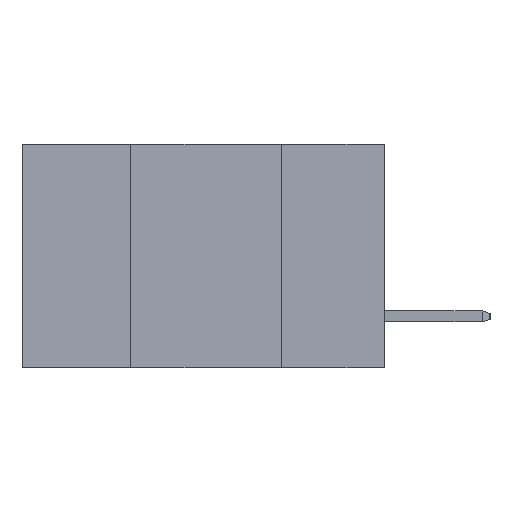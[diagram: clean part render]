
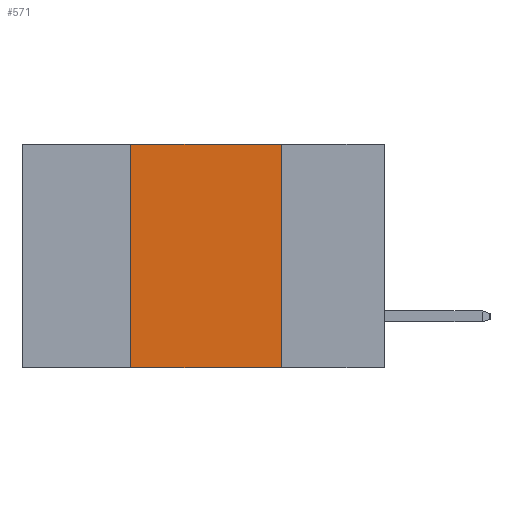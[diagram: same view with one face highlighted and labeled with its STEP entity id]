
A CAD part, left-side view. The second image highlights one B-rep face of the part: STEP entity #571.
In plain terms, the highlighted planar face has unit normal (-1, 0, 0).
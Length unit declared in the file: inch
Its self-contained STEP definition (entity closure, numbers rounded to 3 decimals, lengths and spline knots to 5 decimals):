
#571 = ADVANCED_FACE ( 'NONE', ( #13903 ), #10935, .F. ) ;
#1163 = VECTOR ( 'NONE', #1504, 39.37008 ) ;
#1504 = DIRECTION ( 'NONE',  ( 0., -1., 0. ) ) ;
#1578 = CARTESIAN_POINT ( 'NONE',  ( 0., 0.6, -0.37 ) ) ;
#1893 = DIRECTION ( 'NONE',  ( 0., -1., 0. ) ) ;
#2211 = CARTESIAN_POINT ( 'NONE',  ( 0., 0.17, -0.37 ) ) ;
#2545 = CARTESIAN_POINT ( 'NONE',  ( 0., 0.6, 0. ) ) ;
#3433 = CARTESIAN_POINT ( 'NONE',  ( 0., 0.42, -0.37 ) ) ;
#3455 = DIRECTION ( 'NONE',  ( 0., 0., 1. ) ) ;
#4135 = EDGE_CURVE ( 'NONE', #6457, #13559, #14386, .T. ) ;
#4667 = CARTESIAN_POINT ( 'NONE',  ( 0., 0.42, 0. ) ) ;
#4885 = CARTESIAN_POINT ( 'NONE',  ( 0., 0.6, 0. ) ) ;
#5698 = DIRECTION ( 'NONE',  ( 0., 0., -1. ) ) ;
#5726 = LINE ( 'NONE', #1578, #1163 ) ;
#6457 = VERTEX_POINT ( 'NONE', #4667 ) ;
#6764 = LINE ( 'NONE', #19108, #19841 ) ;
#6936 = VERTEX_POINT ( 'NONE', #18076 ) ;
#7564 = EDGE_LOOP ( 'NONE', ( #8768, #15022, #21575, #13736 ) ) ;
#8113 = EDGE_CURVE ( 'NONE', #6936, #6457, #21948, .T. ) ;
#8383 = DIRECTION ( 'NONE',  ( 1., 0., 0. ) ) ;
#8530 = VECTOR ( 'NONE', #3455, 39.37008 ) ;
#8768 = ORIENTED_EDGE ( 'NONE', *, *, #10841, .F. ) ;
#9779 = VECTOR ( 'NONE', #1893, 39.37008 ) ;
#10447 = EDGE_CURVE ( 'NONE', #6936, #15133, #5726, .T. ) ;
#10841 = EDGE_CURVE ( 'NONE', #13559, #15133, #6764, .T. ) ;
#10935 = PLANE ( 'NONE',  #12965 ) ;
#12965 = AXIS2_PLACEMENT_3D ( 'NONE', #4885, #8383, #5698 ) ;
#13559 = VERTEX_POINT ( 'NONE', #13832 ) ;
#13736 = ORIENTED_EDGE ( 'NONE', *, *, #10447, .T. ) ;
#13832 = CARTESIAN_POINT ( 'NONE',  ( 0., 0.17, 0. ) ) ;
#13903 = FACE_OUTER_BOUND ( 'NONE', #7564, .T. ) ;
#14386 = LINE ( 'NONE', #2545, #9779 ) ;
#15022 = ORIENTED_EDGE ( 'NONE', *, *, #4135, .F. ) ;
#15133 = VERTEX_POINT ( 'NONE', #2211 ) ;
#17627 = DIRECTION ( 'NONE',  ( 0., 0., -1. ) ) ;
#18076 = CARTESIAN_POINT ( 'NONE',  ( 0., 0.42, -0.37 ) ) ;
#19108 = CARTESIAN_POINT ( 'NONE',  ( 0., 0.17, -0.37 ) ) ;
#19841 = VECTOR ( 'NONE', #17627, 39.37008 ) ;
#21575 = ORIENTED_EDGE ( 'NONE', *, *, #8113, .F. ) ;
#21948 = LINE ( 'NONE', #3433, #8530 ) ;
